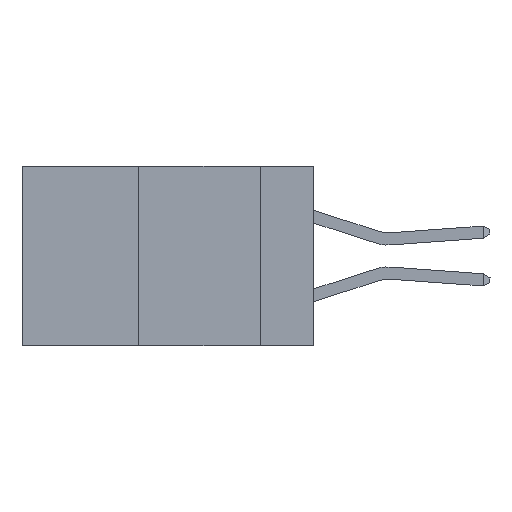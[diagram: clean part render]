
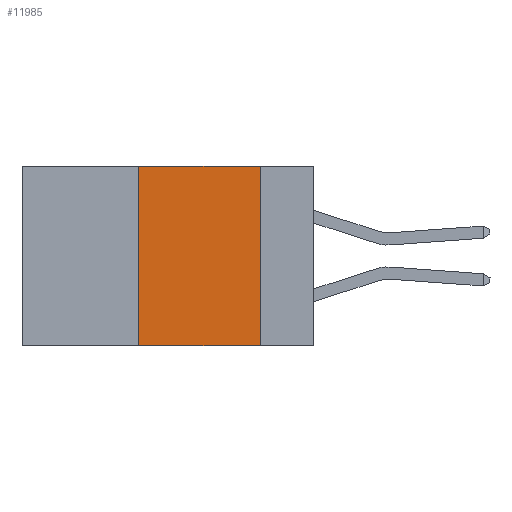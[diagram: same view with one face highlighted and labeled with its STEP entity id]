
A CAD part, left-side view. The second image highlights one B-rep face of the part: STEP entity #11985.
In plain terms, the highlighted planar face has unit normal (-1, 0, 0).
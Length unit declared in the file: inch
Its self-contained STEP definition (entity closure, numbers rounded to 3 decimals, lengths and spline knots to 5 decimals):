
#314 = CARTESIAN_POINT ( 'NONE',  ( 0., 0.6, 0. ) ) ;
#1450 = CARTESIAN_POINT ( 'NONE',  ( 0., 0.36, 0. ) ) ;
#2247 = EDGE_CURVE ( 'NONE', #20988, #13713, #30352, .T. ) ;
#2604 = DIRECTION ( 'NONE',  ( 0., -1., 0. ) ) ;
#3440 = ORIENTED_EDGE ( 'NONE', *, *, #22084, .F. ) ;
#4548 = EDGE_LOOP ( 'NONE', ( #3440, #19217, #14759, #5018 ) ) ;
#5018 = ORIENTED_EDGE ( 'NONE', *, *, #12138, .T. ) ;
#5818 = CARTESIAN_POINT ( 'NONE',  ( 0., 0.36, -0.37 ) ) ;
#6797 = CARTESIAN_POINT ( 'NONE',  ( 0., 0.6, 0. ) ) ;
#7684 = VECTOR ( 'NONE', #2604, 39.37008 ) ;
#10834 = VECTOR ( 'NONE', #28114, 39.37008 ) ;
#11985 = ADVANCED_FACE ( 'NONE', ( #20201 ), #15236, .F. ) ;
#12138 = EDGE_CURVE ( 'NONE', #20988, #27237, #21142, .T. ) ;
#12464 = DIRECTION ( 'NONE',  ( 0., 0., -1. ) ) ;
#13713 = VERTEX_POINT ( 'NONE', #1450 ) ;
#14759 = ORIENTED_EDGE ( 'NONE', *, *, #2247, .F. ) ;
#15171 = CARTESIAN_POINT ( 'NONE',  ( 0., 0.36, 0. ) ) ;
#15236 = PLANE ( 'NONE',  #23319 ) ;
#15470 = VECTOR ( 'NONE', #12464, 39.37008 ) ;
#19217 = ORIENTED_EDGE ( 'NONE', *, *, #19447, .F. ) ;
#19447 = EDGE_CURVE ( 'NONE', #13713, #28354, #26649, .T. ) ;
#19886 = DIRECTION ( 'NONE',  ( 1., 0., 0. ) ) ;
#20201 = FACE_OUTER_BOUND ( 'NONE', #4548, .T. ) ;
#20988 = VERTEX_POINT ( 'NONE', #5818 ) ;
#21142 = LINE ( 'NONE', #21302, #22290 ) ;
#21302 = CARTESIAN_POINT ( 'NONE',  ( 0., 0.6, -0.37 ) ) ;
#22084 = EDGE_CURVE ( 'NONE', #28354, #27237, #22405, .T. ) ;
#22219 = CARTESIAN_POINT ( 'NONE',  ( 0., 0.11, 0. ) ) ;
#22290 = VECTOR ( 'NONE', #31076, 39.37008 ) ;
#22405 = LINE ( 'NONE', #23897, #15470 ) ;
#22686 = CARTESIAN_POINT ( 'NONE',  ( 0., 0.11, -0.37 ) ) ;
#23319 = AXIS2_PLACEMENT_3D ( 'NONE', #314, #19886, #25000 ) ;
#23897 = CARTESIAN_POINT ( 'NONE',  ( 0., 0.11, 0. ) ) ;
#25000 = DIRECTION ( 'NONE',  ( 0., 0., -1. ) ) ;
#26649 = LINE ( 'NONE', #6797, #7684 ) ;
#27237 = VERTEX_POINT ( 'NONE', #22686 ) ;
#28114 = DIRECTION ( 'NONE',  ( 0., 0., 1. ) ) ;
#28354 = VERTEX_POINT ( 'NONE', #22219 ) ;
#30352 = LINE ( 'NONE', #15171, #10834 ) ;
#31076 = DIRECTION ( 'NONE',  ( 0., -1., 0. ) ) ;
